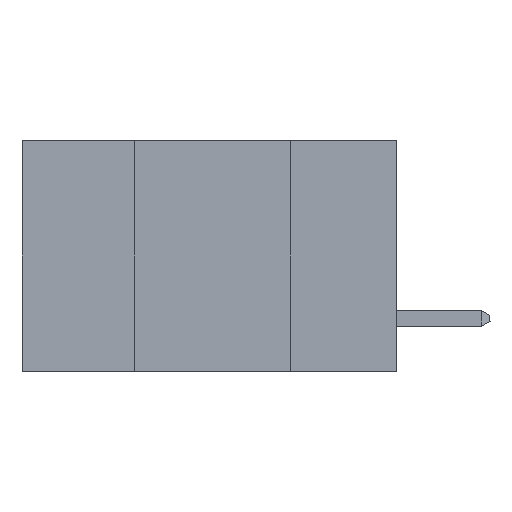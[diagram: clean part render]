
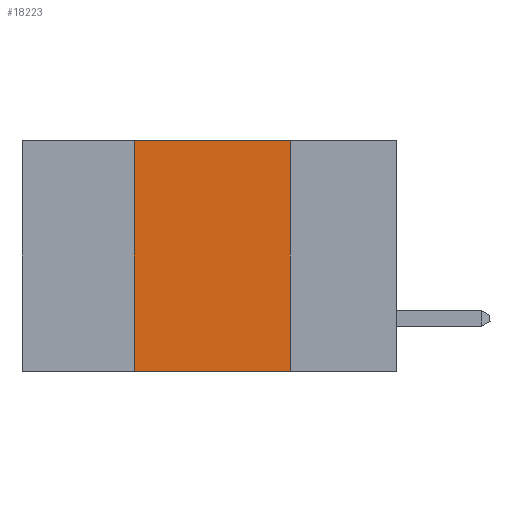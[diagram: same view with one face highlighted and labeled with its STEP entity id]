
A CAD part, left-side view. The second image highlights one B-rep face of the part: STEP entity #18223.
In plain terms, the highlighted planar face has unit normal (-1, 0, 0).
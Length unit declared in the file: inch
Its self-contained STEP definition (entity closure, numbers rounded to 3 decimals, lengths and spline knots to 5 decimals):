
#540 = ORIENTED_EDGE ( 'NONE', *, *, #1614, .F. ) ;
#551 = DIRECTION ( 'NONE',  ( 0., 0., -1. ) ) ;
#611 = CARTESIAN_POINT ( 'NONE',  ( 0., 0.6, 0. ) ) ;
#696 = CARTESIAN_POINT ( 'NONE',  ( 0., 0.17, -0.37 ) ) ;
#1488 = VECTOR ( 'NONE', #12074, 39.37008 ) ;
#1614 = EDGE_CURVE ( 'NONE', #9904, #7555, #6233, .T. ) ;
#2127 = CARTESIAN_POINT ( 'NONE',  ( 0., 0.6, -0.37 ) ) ;
#2495 = CARTESIAN_POINT ( 'NONE',  ( 0., 0.17, 0. ) ) ;
#2793 = LINE ( 'NONE', #3935, #15029 ) ;
#3276 = EDGE_CURVE ( 'NONE', #4119, #7555, #6815, .T. ) ;
#3306 = CARTESIAN_POINT ( 'NONE',  ( 0., 0.6, 0. ) ) ;
#3935 = CARTESIAN_POINT ( 'NONE',  ( 0., 0.42, 0. ) ) ;
#4119 = VERTEX_POINT ( 'NONE', #15654 ) ;
#4807 = CARTESIAN_POINT ( 'NONE',  ( 0., 0.17, 0. ) ) ;
#5094 = DIRECTION ( 'NONE',  ( 0., 0., -1. ) ) ;
#6233 = LINE ( 'NONE', #4807, #9976 ) ;
#6815 = LINE ( 'NONE', #2127, #1488 ) ;
#7094 = VECTOR ( 'NONE', #13532, 39.37008 ) ;
#7555 = VERTEX_POINT ( 'NONE', #696 ) ;
#8128 = EDGE_CURVE ( 'NONE', #12390, #9904, #15330, .T. ) ;
#9628 = EDGE_CURVE ( 'NONE', #4119, #12390, #2793, .T. ) ;
#9904 = VERTEX_POINT ( 'NONE', #2495 ) ;
#9976 = VECTOR ( 'NONE', #551, 39.37008 ) ;
#11038 = ORIENTED_EDGE ( 'NONE', *, *, #9628, .F. ) ;
#11235 = ORIENTED_EDGE ( 'NONE', *, *, #8128, .F. ) ;
#12074 = DIRECTION ( 'NONE',  ( 0., -1., 0. ) ) ;
#12390 = VERTEX_POINT ( 'NONE', #15090 ) ;
#13231 = DIRECTION ( 'NONE',  ( 1., 0., 0. ) ) ;
#13240 = EDGE_LOOP ( 'NONE', ( #540, #11235, #11038, #15774 ) ) ;
#13532 = DIRECTION ( 'NONE',  ( 0., -1., 0. ) ) ;
#15029 = VECTOR ( 'NONE', #16495, 39.37008 ) ;
#15090 = CARTESIAN_POINT ( 'NONE',  ( 0., 0.42, 0. ) ) ;
#15330 = LINE ( 'NONE', #611, #7094 ) ;
#15654 = CARTESIAN_POINT ( 'NONE',  ( 0., 0.42, -0.37 ) ) ;
#15774 = ORIENTED_EDGE ( 'NONE', *, *, #3276, .T. ) ;
#16495 = DIRECTION ( 'NONE',  ( 0., 0., 1. ) ) ;
#16503 = FACE_OUTER_BOUND ( 'NONE', #13240, .T. ) ;
#17544 = AXIS2_PLACEMENT_3D ( 'NONE', #3306, #13231, #5094 ) ;
#17780 = PLANE ( 'NONE',  #17544 ) ;
#18223 = ADVANCED_FACE ( 'NONE', ( #16503 ), #17780, .F. ) ;
